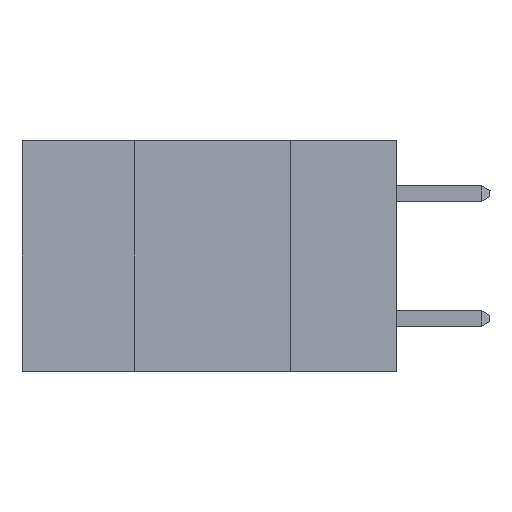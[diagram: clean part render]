
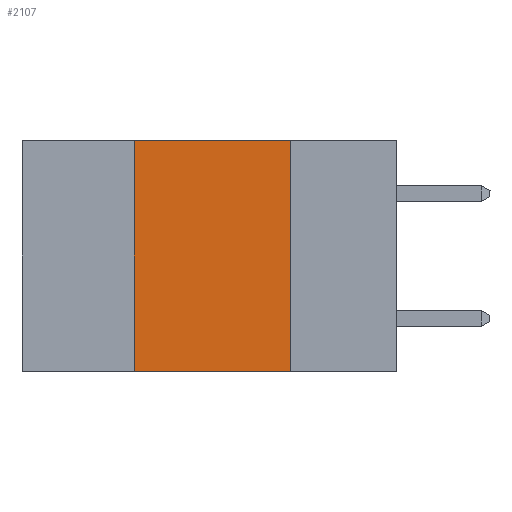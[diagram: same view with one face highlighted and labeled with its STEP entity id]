
A CAD part, left-side view. The second image highlights one B-rep face of the part: STEP entity #2107.
In plain terms, the highlighted planar face has unit normal (-1, 0, 0).
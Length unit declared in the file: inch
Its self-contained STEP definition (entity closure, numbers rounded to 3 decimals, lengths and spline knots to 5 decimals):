
#322 = DIRECTION ( 'NONE',  ( 1., 0., 0. ) ) ;
#854 = ORIENTED_EDGE ( 'NONE', *, *, #7171, .T. ) ;
#1192 = LINE ( 'NONE', #7652, #5998 ) ;
#1414 = EDGE_CURVE ( 'NONE', #10347, #11377, #9632, .T. ) ;
#1990 = EDGE_CURVE ( 'NONE', #11377, #9315, #1192, .T. ) ;
#2107 = ADVANCED_FACE ( 'NONE', ( #11791 ), #7972, .F. ) ;
#2424 = DIRECTION ( 'NONE',  ( 0., 0., 1. ) ) ;
#3333 = DIRECTION ( 'NONE',  ( 0., -1., 0. ) ) ;
#3686 = ORIENTED_EDGE ( 'NONE', *, *, #7414, .F. ) ;
#5871 = CARTESIAN_POINT ( 'NONE',  ( 0., 0.17, -0.37 ) ) ;
#5998 = VECTOR ( 'NONE', #6231, 39.37008 ) ;
#6231 = DIRECTION ( 'NONE',  ( 0., 0., -1. ) ) ;
#6292 = EDGE_LOOP ( 'NONE', ( #9925, #6657, #3686, #854 ) ) ;
#6458 = AXIS2_PLACEMENT_3D ( 'NONE', #7959, #322, #9516 ) ;
#6462 = VERTEX_POINT ( 'NONE', #6986 ) ;
#6657 = ORIENTED_EDGE ( 'NONE', *, *, #1414, .F. ) ;
#6828 = DIRECTION ( 'NONE',  ( 0., -1., 0. ) ) ;
#6986 = CARTESIAN_POINT ( 'NONE',  ( 0., 0.42, -0.37 ) ) ;
#7071 = LINE ( 'NONE', #7666, #11541 ) ;
#7171 = EDGE_CURVE ( 'NONE', #6462, #9315, #7071, .T. ) ;
#7221 = VECTOR ( 'NONE', #3333, 39.37008 ) ;
#7414 = EDGE_CURVE ( 'NONE', #6462, #10347, #11668, .T. ) ;
#7652 = CARTESIAN_POINT ( 'NONE',  ( 0., 0.17, 0. ) ) ;
#7666 = CARTESIAN_POINT ( 'NONE',  ( 0., 0.6, -0.37 ) ) ;
#7959 = CARTESIAN_POINT ( 'NONE',  ( 0., 0.6, 0. ) ) ;
#7972 = PLANE ( 'NONE',  #6458 ) ;
#8032 = CARTESIAN_POINT ( 'NONE',  ( 0., 0.6, 0. ) ) ;
#9208 = CARTESIAN_POINT ( 'NONE',  ( 0., 0.42, 0. ) ) ;
#9315 = VERTEX_POINT ( 'NONE', #5871 ) ;
#9516 = DIRECTION ( 'NONE',  ( 0., 0., -1. ) ) ;
#9632 = LINE ( 'NONE', #8032, #7221 ) ;
#9925 = ORIENTED_EDGE ( 'NONE', *, *, #1990, .F. ) ;
#10347 = VERTEX_POINT ( 'NONE', #11912 ) ;
#10685 = CARTESIAN_POINT ( 'NONE',  ( 0., 0.17, 0. ) ) ;
#11116 = VECTOR ( 'NONE', #2424, 39.37008 ) ;
#11377 = VERTEX_POINT ( 'NONE', #10685 ) ;
#11541 = VECTOR ( 'NONE', #6828, 39.37008 ) ;
#11668 = LINE ( 'NONE', #9208, #11116 ) ;
#11791 = FACE_OUTER_BOUND ( 'NONE', #6292, .T. ) ;
#11912 = CARTESIAN_POINT ( 'NONE',  ( 0., 0.42, 0. ) ) ;
